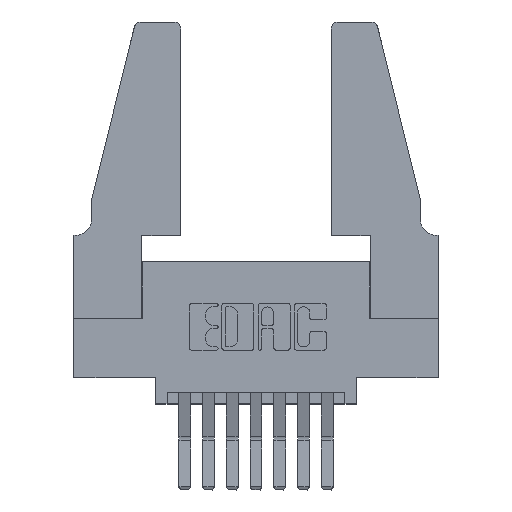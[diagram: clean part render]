
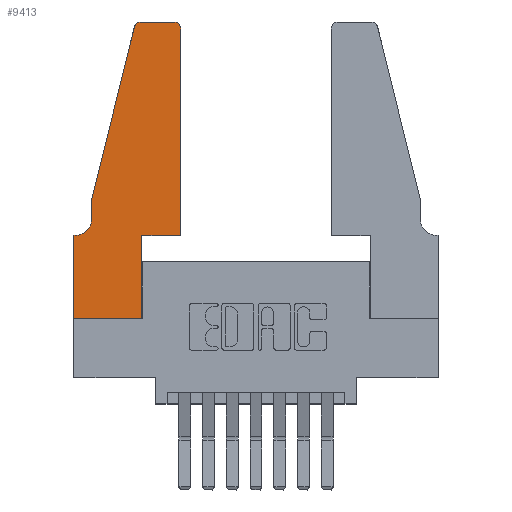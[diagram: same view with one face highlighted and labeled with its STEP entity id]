
A CAD part, top view. The second image highlights one B-rep face of the part: STEP entity #9413.
In plain terms, the highlighted planar face has unit normal (0, 0, 1).
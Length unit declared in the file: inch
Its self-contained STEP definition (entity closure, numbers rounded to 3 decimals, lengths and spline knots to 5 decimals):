
#4 = LINE ( 'NONE', #7923, #2876 ) ;
#265 = ORIENTED_EDGE ( 'NONE', *, *, #7485, .T. ) ;
#266 = VERTEX_POINT ( 'NONE', #9901 ) ;
#988 = DIRECTION ( 'NONE',  ( 0., -1., 0. ) ) ;
#1001 = CARTESIAN_POINT ( 'NONE',  ( 0.2865, 0.35, 0.37 ) ) ;
#1323 = CARTESIAN_POINT ( 'NONE',  ( 0.4505, 0.35, 0.37 ) ) ;
#1461 = CARTESIAN_POINT ( 'NONE',  ( 0.284, 1.25, 0.37 ) ) ;
#1496 = VERTEX_POINT ( 'NONE', #5751 ) ;
#1639 = VECTOR ( 'NONE', #4350, 39.37008 ) ;
#1654 = VECTOR ( 'NONE', #9151, 39.37008 ) ;
#1987 = LINE ( 'NONE', #1001, #11542 ) ;
#2149 = ORIENTED_EDGE ( 'NONE', *, *, #2234, .T. ) ;
#2231 = VERTEX_POINT ( 'NONE', #3399 ) ;
#2233 = VECTOR ( 'NONE', #988, 39.37008 ) ;
#2234 = EDGE_CURVE ( 'NONE', #5937, #5123, #4378, .T. ) ;
#2239 = VERTEX_POINT ( 'NONE', #4339 ) ;
#2358 = CARTESIAN_POINT ( 'NONE',  ( 0., 0., 0.37 ) ) ;
#2442 = VERTEX_POINT ( 'NONE', #4203 ) ;
#2449 = LINE ( 'NONE', #7635, #6729 ) ;
#2508 = VERTEX_POINT ( 'NONE', #1323 ) ;
#2522 = CARTESIAN_POINT ( 'NONE',  ( 0.0755, 0.42, 0.37 ) ) ;
#2568 = LINE ( 'NONE', #3109, #2233 ) ;
#2876 = VECTOR ( 'NONE', #5053, 39.37008 ) ;
#3033 = DIRECTION ( 'NONE',  ( 1., 0., 0. ) ) ;
#3109 = CARTESIAN_POINT ( 'NONE',  ( 0.0755, 0.5, 0.37 ) ) ;
#3172 = CIRCLE ( 'NONE', #7307, 0.03 ) ;
#3346 = VERTEX_POINT ( 'NONE', #4316 ) ;
#3399 = CARTESIAN_POINT ( 'NONE',  ( 0.4505, 1.22, 0.37 ) ) ;
#3739 = DIRECTION ( 'NONE',  ( -1., 0., 0. ) ) ;
#4203 = CARTESIAN_POINT ( 'NONE',  ( 0., 0.35, 0.37 ) ) ;
#4248 = AXIS2_PLACEMENT_3D ( 'NONE', #11151, #12096, #6545 ) ;
#4253 = ORIENTED_EDGE ( 'NONE', *, *, #10113, .T. ) ;
#4316 = CARTESIAN_POINT ( 'NONE',  ( 0.0055, 0.35, 0.37 ) ) ;
#4339 = CARTESIAN_POINT ( 'NONE',  ( 0.4205, 1.25, 0.37 ) ) ;
#4350 = DIRECTION ( 'NONE',  ( 1., 0., 0. ) ) ;
#4378 = LINE ( 'NONE', #2358, #1639 ) ;
#4572 = LINE ( 'NONE', #8138, #9286 ) ;
#4632 = PLANE ( 'NONE',  #4248 ) ;
#4741 = CARTESIAN_POINT ( 'NONE',  ( 0.2605, 1.25, 0.37 ) ) ;
#4916 = CARTESIAN_POINT ( 'NONE',  ( 0.4205, 1.22, 0.37 ) ) ;
#4941 = VECTOR ( 'NONE', #3739, 39.37008 ) ;
#5053 = DIRECTION ( 'NONE',  ( 0., -1., 0. ) ) ;
#5067 = ORIENTED_EDGE ( 'NONE', *, *, #8584, .T. ) ;
#5105 = CARTESIAN_POINT ( 'NONE',  ( 0.284, 1.22, 0.37 ) ) ;
#5123 = VERTEX_POINT ( 'NONE', #12341 ) ;
#5292 = ORIENTED_EDGE ( 'NONE', *, *, #8142, .T. ) ;
#5327 = CARTESIAN_POINT ( 'NONE',  ( 0.0055, 0.42, 0.37 ) ) ;
#5340 = DIRECTION ( 'NONE',  ( 1., 0., 0. ) ) ;
#5527 = EDGE_LOOP ( 'NONE', ( #7251, #9502, #5292, #7429, #9229, #265, #11773, #2149, #5067, #11373, #4253, #5721 ) ) ;
#5620 = EDGE_CURVE ( 'NONE', #2231, #2239, #3172, .T. ) ;
#5694 = EDGE_CURVE ( 'NONE', #7582, #3346, #9894, .T. ) ;
#5721 = ORIENTED_EDGE ( 'NONE', *, *, #5620, .T. ) ;
#5751 = CARTESIAN_POINT ( 'NONE',  ( 0.0755, 0.5, 0.37 ) ) ;
#5836 = VECTOR ( 'NONE', #3033, 39.37008 ) ;
#5937 = VERTEX_POINT ( 'NONE', #7728 ) ;
#6029 = EDGE_CURVE ( 'NONE', #266, #2508, #8300, .T. ) ;
#6058 = DIRECTION ( 'NONE',  ( 1., 0., 0. ) ) ;
#6064 = EDGE_CURVE ( 'NONE', #2442, #5937, #4, .T. ) ;
#6259 = DIRECTION ( 'NONE',  ( -1., 0., 0. ) ) ;
#6545 = DIRECTION ( 'NONE',  ( 1., 0., 0. ) ) ;
#6729 = VECTOR ( 'NONE', #12244, 39.37008 ) ;
#7251 = ORIENTED_EDGE ( 'NONE', *, *, #11315, .T. ) ;
#7307 = AXIS2_PLACEMENT_3D ( 'NONE', #4916, #11429, #5340 ) ;
#7429 = ORIENTED_EDGE ( 'NONE', *, *, #12214, .T. ) ;
#7485 = EDGE_CURVE ( 'NONE', #3346, #2442, #4572, .T. ) ;
#7582 = VERTEX_POINT ( 'NONE', #2522 ) ;
#7606 = VERTEX_POINT ( 'NONE', #1461 ) ;
#7635 = CARTESIAN_POINT ( 'NONE',  ( 0.4505, 0.35, 0.37 ) ) ;
#7718 = CIRCLE ( 'NONE', #11558, 0.03 ) ;
#7728 = CARTESIAN_POINT ( 'NONE',  ( 0., 0., 0.37 ) ) ;
#7883 = VERTEX_POINT ( 'NONE', #11471 ) ;
#7923 = CARTESIAN_POINT ( 'NONE',  ( 0., 0., 0.37 ) ) ;
#8138 = CARTESIAN_POINT ( 'NONE',  ( 0.0755, 0.35, 0.37 ) ) ;
#8142 = EDGE_CURVE ( 'NONE', #7883, #1496, #9414, .T. ) ;
#8300 = LINE ( 'NONE', #12458, #5836 ) ;
#8584 = EDGE_CURVE ( 'NONE', #5123, #266, #1987, .T. ) ;
#8893 = DIRECTION ( 'NONE',  ( 0., 1., 0. ) ) ;
#9151 = DIRECTION ( 'NONE',  ( -0.239, -0.971, 0. ) ) ;
#9229 = ORIENTED_EDGE ( 'NONE', *, *, #5694, .T. ) ;
#9286 = VECTOR ( 'NONE', #10001, 39.37008 ) ;
#9413 = ADVANCED_FACE ( 'NONE', ( #12117 ), #4632, .T. ) ;
#9414 = LINE ( 'NONE', #10069, #1654 ) ;
#9502 = ORIENTED_EDGE ( 'NONE', *, *, #12190, .T. ) ;
#9894 = CIRCLE ( 'NONE', #11636, 0.07 ) ;
#9901 = CARTESIAN_POINT ( 'NONE',  ( 0.2865, 0.35, 0.37 ) ) ;
#10001 = DIRECTION ( 'NONE',  ( -1., 0., 0. ) ) ;
#10069 = CARTESIAN_POINT ( 'NONE',  ( 0.0755, 0.5, 0.37 ) ) ;
#10113 = EDGE_CURVE ( 'NONE', #2508, #2231, #2449, .T. ) ;
#10203 = LINE ( 'NONE', #4741, #4941 ) ;
#11151 = CARTESIAN_POINT ( 'NONE',  ( 0., 0.35, 0.37 ) ) ;
#11315 = EDGE_CURVE ( 'NONE', #2239, #7606, #10203, .T. ) ;
#11373 = ORIENTED_EDGE ( 'NONE', *, *, #6029, .T. ) ;
#11429 = DIRECTION ( 'NONE',  ( 0., 0., 1. ) ) ;
#11471 = CARTESIAN_POINT ( 'NONE',  ( 0.25487, 1.22718, 0.37 ) ) ;
#11542 = VECTOR ( 'NONE', #8893, 39.37008 ) ;
#11558 = AXIS2_PLACEMENT_3D ( 'NONE', #5105, #11593, #6058 ) ;
#11593 = DIRECTION ( 'NONE',  ( 0., 0., 1. ) ) ;
#11636 = AXIS2_PLACEMENT_3D ( 'NONE', #5327, #11803, #6259 ) ;
#11773 = ORIENTED_EDGE ( 'NONE', *, *, #6064, .T. ) ;
#11803 = DIRECTION ( 'NONE',  ( 0., 0., -1. ) ) ;
#12096 = DIRECTION ( 'NONE',  ( 0., 0., 1. ) ) ;
#12117 = FACE_OUTER_BOUND ( 'NONE', #5527, .T. ) ;
#12190 = EDGE_CURVE ( 'NONE', #7606, #7883, #7718, .T. ) ;
#12214 = EDGE_CURVE ( 'NONE', #1496, #7582, #2568, .T. ) ;
#12244 = DIRECTION ( 'NONE',  ( 0., 1., 0. ) ) ;
#12341 = CARTESIAN_POINT ( 'NONE',  ( 0.2865, 0., 0.37 ) ) ;
#12458 = CARTESIAN_POINT ( 'NONE',  ( 0.4505, 0.35, 0.37 ) ) ;
